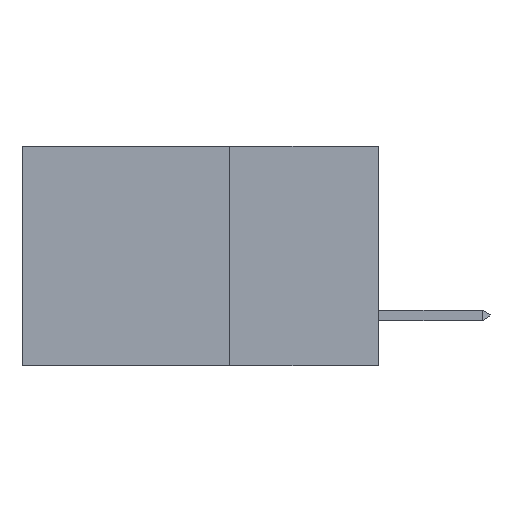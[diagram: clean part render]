
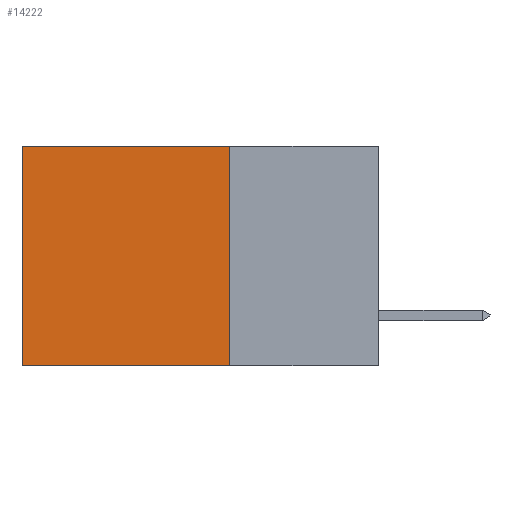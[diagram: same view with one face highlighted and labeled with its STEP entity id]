
A CAD part, left-side view. The second image highlights one B-rep face of the part: STEP entity #14222.
In plain terms, the highlighted planar face has unit normal (-1, 0, 0).
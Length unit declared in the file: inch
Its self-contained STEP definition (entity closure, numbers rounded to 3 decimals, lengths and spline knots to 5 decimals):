
#449 = AXIS2_PLACEMENT_3D ( 'NONE', #7221, #5988, #7500 ) ;
#797 = VECTOR ( 'NONE', #6042, 39.37008 ) ;
#955 = CARTESIAN_POINT ( 'NONE',  ( 0.2615, 0.6, 0. ) ) ;
#2068 = CARTESIAN_POINT ( 'NONE',  ( 0.2615, 0.25, -0.37 ) ) ;
#2308 = CARTESIAN_POINT ( 'NONE',  ( 0.2615, 0.25, 0. ) ) ;
#2854 = EDGE_CURVE ( 'NONE', #14054, #15294, #3436, .T. ) ;
#3436 = LINE ( 'NONE', #7442, #13922 ) ;
#3725 = VERTEX_POINT ( 'NONE', #2068 ) ;
#4297 = ORIENTED_EDGE ( 'NONE', *, *, #2854, .T. ) ;
#4473 = CARTESIAN_POINT ( 'NONE',  ( 0.2615, 0.25, -0.37 ) ) ;
#4649 = DIRECTION ( 'NONE',  ( 0., 0., -1. ) ) ;
#5988 = DIRECTION ( 'NONE',  ( 1., 0., 0. ) ) ;
#6042 = DIRECTION ( 'NONE',  ( 0., 1., 0. ) ) ;
#6306 = VERTEX_POINT ( 'NONE', #14571 ) ;
#7046 = LINE ( 'NONE', #10883, #797 ) ;
#7221 = CARTESIAN_POINT ( 'NONE',  ( 0.2615, 0.25, -0.37 ) ) ;
#7442 = CARTESIAN_POINT ( 'NONE',  ( 0.2615, 0.25, 0. ) ) ;
#7500 = DIRECTION ( 'NONE',  ( 0., 0., -1. ) ) ;
#7792 = EDGE_CURVE ( 'NONE', #14054, #3725, #11417, .T. ) ;
#8351 = VECTOR ( 'NONE', #4649, 39.37008 ) ;
#9213 = EDGE_LOOP ( 'NONE', ( #16589, #10018, #16895, #4297 ) ) ;
#9906 = FACE_OUTER_BOUND ( 'NONE', #9213, .T. ) ;
#10018 = ORIENTED_EDGE ( 'NONE', *, *, #10146, .F. ) ;
#10146 = EDGE_CURVE ( 'NONE', #3725, #6306, #7046, .T. ) ;
#10750 = CARTESIAN_POINT ( 'NONE',  ( 0.2615, 0.6, -0.37 ) ) ;
#10883 = CARTESIAN_POINT ( 'NONE',  ( 0.2615, 0.25, -0.37 ) ) ;
#11417 = LINE ( 'NONE', #4473, #8351 ) ;
#11530 = DIRECTION ( 'NONE',  ( 0., 1., 0. ) ) ;
#12163 = DIRECTION ( 'NONE',  ( 0., 0., -1. ) ) ;
#12257 = LINE ( 'NONE', #10750, #12420 ) ;
#12420 = VECTOR ( 'NONE', #12163, 39.37008 ) ;
#13922 = VECTOR ( 'NONE', #11530, 39.37008 ) ;
#14054 = VERTEX_POINT ( 'NONE', #2308 ) ;
#14222 = ADVANCED_FACE ( 'NONE', ( #9906 ), #17034, .F. ) ;
#14571 = CARTESIAN_POINT ( 'NONE',  ( 0.2615, 0.6, -0.37 ) ) ;
#15294 = VERTEX_POINT ( 'NONE', #955 ) ;
#16589 = ORIENTED_EDGE ( 'NONE', *, *, #16820, .T. ) ;
#16820 = EDGE_CURVE ( 'NONE', #15294, #6306, #12257, .T. ) ;
#16895 = ORIENTED_EDGE ( 'NONE', *, *, #7792, .F. ) ;
#17034 = PLANE ( 'NONE',  #449 ) ;
